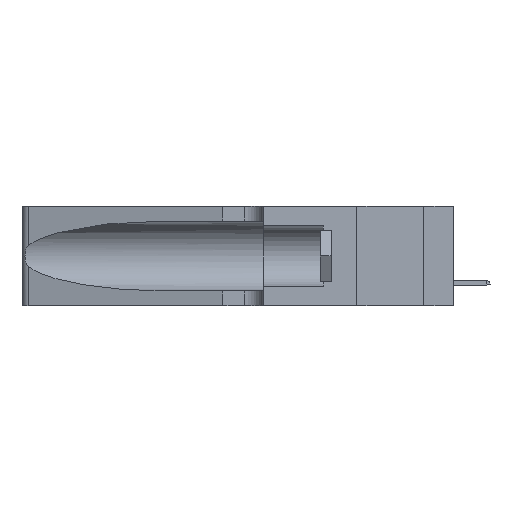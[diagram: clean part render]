
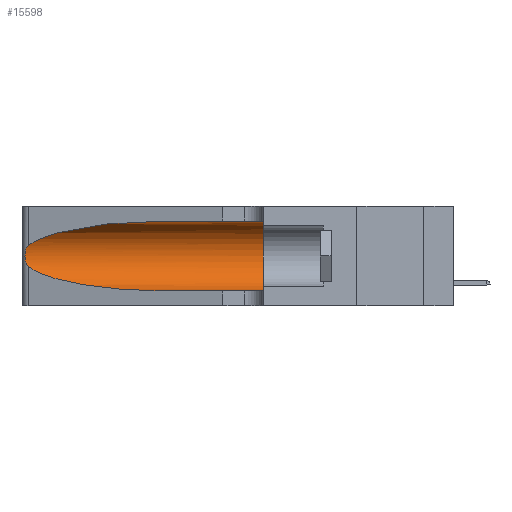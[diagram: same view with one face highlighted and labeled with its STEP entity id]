
A CAD part, left-side view. The second image highlights one B-rep face of the part: STEP entity #15598.
In plain terms, the highlighted cylindrical face has radius 3.308 mm (diameter 6.617 mm), a partial arc.
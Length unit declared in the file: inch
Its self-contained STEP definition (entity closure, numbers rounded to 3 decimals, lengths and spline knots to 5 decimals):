
#108 = CARTESIAN_POINT ( 'NONE',  ( 0.25789, 1.23486, 0.15765 ) ) ;
#200 = EDGE_CURVE ( 'NONE', #4065, #1824, #39720, .T. ) ;
#442 = CARTESIAN_POINT ( 'NONE',  ( 0.1305, 1.61858, 0.185 ) ) ;
#608 = B_SPLINE_CURVE_WITH_KNOTS ( 'NONE', 3,
 ( #35482, #35712, #17681, #17914, #38947, #45683, #17461, #32229, #14000, #20932, #108, #10755, #28088, #32015 ),
 .UNSPECIFIED., .F., .F.,
 ( 4, 2, 2, 2, 2, 2, 4 ),
 ( 0., 0.00027, 0.00053, 0.00107, 0.0016, 0.00187, 0.00214 ),
 .UNSPECIFIED. ) ;
#811 = DIRECTION ( 'NONE',  ( 0., -1., 0. ) ) ;
#1481 = CARTESIAN_POINT ( 'NONE',  ( 0.18966, 0.96281, 0.31525 ) ) ;
#1824 = VERTEX_POINT ( 'NONE', #44364 ) ;
#3759 = ORIENTED_EDGE ( 'NONE', *, *, #15149, .T. ) ;
#4065 = VERTEX_POINT ( 'NONE', #13036 ) ;
#4497 = ORIENTED_EDGE ( 'NONE', *, *, #23021, .T. ) ;
#4498 = CARTESIAN_POINT ( 'NONE',  ( 0.1305, 0.72297, 0.31525 ) ) ;
#5619 = CARTESIAN_POINT ( 'NONE',  ( 0.1305, 0.72297, 0.05475 ) ) ;
#6488 = DIRECTION ( 'NONE',  ( 0., 0., 1. ) ) ;
#6629 = VERTEX_POINT ( 'NONE', #43862 ) ;
#7175 = FACE_OUTER_BOUND ( 'NONE', #17004, .T. ) ;
#10755 = CARTESIAN_POINT ( 'NONE',  ( 0.25639, 1.23186, 0.15144 ) ) ;
#11196 = VERTEX_POINT ( 'NONE', #12641 ) ;
#12337 = VERTEX_POINT ( 'NONE', #5619 ) ;
#12466 = LINE ( 'NONE', #25872, #44833 ) ;
#12641 = CARTESIAN_POINT ( 'NONE',  ( 0.25487, 1.22718, 0.14631 ) ) ;
#13036 = CARTESIAN_POINT ( 'NONE',  ( 0.1305, 0.35, 0.31525 ) ) ;
#14000 = CARTESIAN_POINT ( 'NONE',  ( 0.26017, 1.23833, 0.17102 ) ) ;
#14335 = DIRECTION ( 'NONE',  ( 0., -1., 0. ) ) ;
#15149 = EDGE_CURVE ( 'NONE', #6629, #11196, #608, .T. ) ;
#15598 = ADVANCED_FACE ( 'NONE', ( #7175 ), #17571, .F. ) ;
#16856 = AXIS2_PLACEMENT_3D ( 'NONE', #24727, #31216, #6488 ) ;
#17004 = EDGE_LOOP ( 'NONE', ( #30519, #3759, #42558, #4497, #21653, #38454 ) ) ;
#17461 = CARTESIAN_POINT ( 'NONE',  ( 0.26075, 1.23896, 0.19203 ) ) ;
#17482 = LINE ( 'NONE', #17708, #45485 ) ;
#17571 = CYLINDRICAL_SURFACE ( 'NONE', #38622, 0.13025 ) ;
#17681 = CARTESIAN_POINT ( 'NONE',  ( 0.25639, 1.23184, 0.21858 ) ) ;
#17708 = CARTESIAN_POINT ( 'NONE',  ( 0.1305, 1.61858, 0.31525 ) ) ;
#17914 = CARTESIAN_POINT ( 'NONE',  ( 0.25787, 1.23484, 0.2124 ) ) ;
#20932 = CARTESIAN_POINT ( 'NONE',  ( 0.25856, 1.23593, 0.16098 ) ) ;
#21653 = ORIENTED_EDGE ( 'NONE', *, *, #200, .F. ) ;
#21915 =( BOUNDED_CURVE ( )  B_SPLINE_CURVE ( 3, ( #4498, #1481, #32915, #33611 ),
 .UNSPECIFIED., .F., .F. ) 
 B_SPLINE_CURVE_WITH_KNOTS ( ( 4, 4 ),
 ( 1.5708, 2.84003 ),
 .UNSPECIFIED. ) 
 CURVE ( )  GEOMETRIC_REPRESENTATION_ITEM ( )  RATIONAL_B_SPLINE_CURVE ( ( 1., 0.87, 0.87, 1. ) ) 
 REPRESENTATION_ITEM ( '' )  );
#23021 = EDGE_CURVE ( 'NONE', #12337, #1824, #12466, .T. ) ;
#24563 = EDGE_CURVE ( 'NONE', #44113, #4065, #17482, .T. ) ;
#24727 = CARTESIAN_POINT ( 'NONE',  ( 0.1305, 0.35, 0.185 ) ) ;
#25872 = CARTESIAN_POINT ( 'NONE',  ( 0.1305, 1.61858, 0.05475 ) ) ;
#27055 = CARTESIAN_POINT ( 'NONE',  ( 0.18966, 0.96281, 0.05475 ) ) ;
#28088 = CARTESIAN_POINT ( 'NONE',  ( 0.25555, 1.22993, 0.14849 ) ) ;
#29691 = CARTESIAN_POINT ( 'NONE',  ( 0.1305, 0.72297, 0.31525 ) ) ;
#30519 = ORIENTED_EDGE ( 'NONE', *, *, #42880, .T. ) ;
#31216 = DIRECTION ( 'NONE',  ( 0., 1., 0. ) ) ;
#32015 = CARTESIAN_POINT ( 'NONE',  ( 0.25487, 1.22718, 0.14631 ) ) ;
#32229 = CARTESIAN_POINT ( 'NONE',  ( 0.26075, 1.23896, 0.178 ) ) ;
#32572 = DIRECTION ( 'NONE',  ( 0., 0., -1. ) ) ;
#32915 = CARTESIAN_POINT ( 'NONE',  ( 0.2373, 1.15595, 0.28018 ) ) ;
#33611 = CARTESIAN_POINT ( 'NONE',  ( 0.25487, 1.22718, 0.22369 ) ) ;
#34358 =( BOUNDED_CURVE ( )  B_SPLINE_CURVE ( 3, ( #34682, #37924, #27055, #41626 ),
 .UNSPECIFIED., .F., .F. ) 
 B_SPLINE_CURVE_WITH_KNOTS ( ( 4, 4 ),
 ( 3.44316, 4.71239 ),
 .UNSPECIFIED. ) 
 CURVE ( )  GEOMETRIC_REPRESENTATION_ITEM ( )  RATIONAL_B_SPLINE_CURVE ( ( 1., 0.87, 0.87, 1. ) ) 
 REPRESENTATION_ITEM ( '' )  );
#34682 = CARTESIAN_POINT ( 'NONE',  ( 0.25487, 1.22718, 0.14631 ) ) ;
#35482 = CARTESIAN_POINT ( 'NONE',  ( 0.25487, 1.22718, 0.22369 ) ) ;
#35712 = CARTESIAN_POINT ( 'NONE',  ( 0.25555, 1.22994, 0.2215 ) ) ;
#37924 = CARTESIAN_POINT ( 'NONE',  ( 0.2373, 1.15595, 0.08982 ) ) ;
#38454 = ORIENTED_EDGE ( 'NONE', *, *, #24563, .F. ) ;
#38622 = AXIS2_PLACEMENT_3D ( 'NONE', #442, #14335, #32572 ) ;
#38947 = CARTESIAN_POINT ( 'NONE',  ( 0.25854, 1.2359, 0.20912 ) ) ;
#39720 = CIRCLE ( 'NONE', #16856, 0.13025 ) ;
#40210 = DIRECTION ( 'NONE',  ( 0., -1., 0. ) ) ;
#40511 = EDGE_CURVE ( 'NONE', #11196, #12337, #34358, .T. ) ;
#41626 = CARTESIAN_POINT ( 'NONE',  ( 0.1305, 0.72297, 0.05475 ) ) ;
#42558 = ORIENTED_EDGE ( 'NONE', *, *, #40511, .T. ) ;
#42880 = EDGE_CURVE ( 'NONE', #44113, #6629, #21915, .T. ) ;
#43862 = CARTESIAN_POINT ( 'NONE',  ( 0.25487, 1.22718, 0.22369 ) ) ;
#44113 = VERTEX_POINT ( 'NONE', #29691 ) ;
#44364 = CARTESIAN_POINT ( 'NONE',  ( 0.1305, 0.35, 0.05475 ) ) ;
#44833 = VECTOR ( 'NONE', #40210, 39.37008 ) ;
#45485 = VECTOR ( 'NONE', #811, 39.37008 ) ;
#45683 = CARTESIAN_POINT ( 'NONE',  ( 0.26018, 1.23835, 0.19895 ) ) ;
